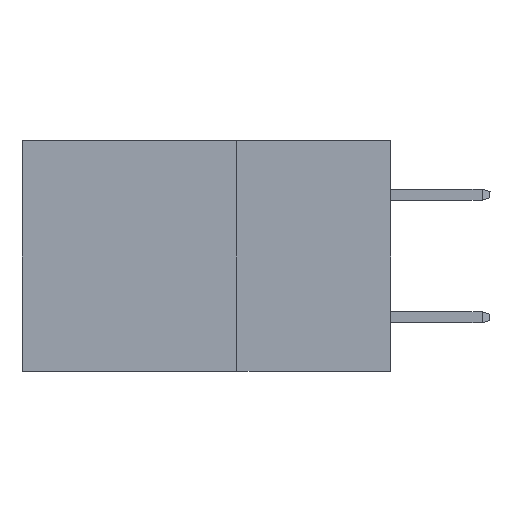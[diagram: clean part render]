
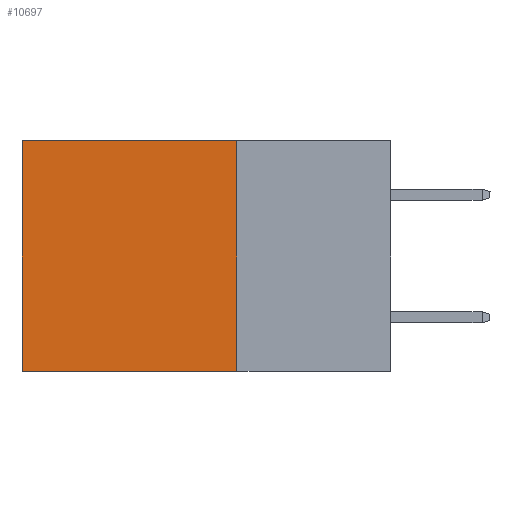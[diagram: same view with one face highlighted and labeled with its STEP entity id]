
A CAD part, left-side view. The second image highlights one B-rep face of the part: STEP entity #10697.
In plain terms, the highlighted planar face has unit normal (-1, 0, 0).
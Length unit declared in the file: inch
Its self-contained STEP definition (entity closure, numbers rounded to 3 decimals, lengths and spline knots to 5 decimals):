
#198 = CARTESIAN_POINT ( 'NONE',  ( 0.2875, 0.6, 0. ) ) ;
#1148 = EDGE_LOOP ( 'NONE', ( #4128, #6292, #8601, #3034 ) ) ;
#2045 = CARTESIAN_POINT ( 'NONE',  ( 0.2875, 0.25, -0.375 ) ) ;
#2134 = AXIS2_PLACEMENT_3D ( 'NONE', #2045, #3228, #10731 ) ;
#3034 = ORIENTED_EDGE ( 'NONE', *, *, #6800, .T. ) ;
#3228 = DIRECTION ( 'NONE',  ( 1., 0., 0. ) ) ;
#3261 = VERTEX_POINT ( 'NONE', #7658 ) ;
#3534 = DIRECTION ( 'NONE',  ( 0., 0., -1. ) ) ;
#3937 = EDGE_CURVE ( 'NONE', #3261, #6011, #5675, .T. ) ;
#4128 = ORIENTED_EDGE ( 'NONE', *, *, #8604, .T. ) ;
#4240 = CARTESIAN_POINT ( 'NONE',  ( 0.2875, 0.25, -0.375 ) ) ;
#4877 = VECTOR ( 'NONE', #5059, 39.37008 ) ;
#5059 = DIRECTION ( 'NONE',  ( 0., 1., 0. ) ) ;
#5675 = LINE ( 'NONE', #11109, #6325 ) ;
#6011 = VERTEX_POINT ( 'NONE', #12541 ) ;
#6292 = ORIENTED_EDGE ( 'NONE', *, *, #11213, .F. ) ;
#6325 = VECTOR ( 'NONE', #12013, 39.37008 ) ;
#6518 = VERTEX_POINT ( 'NONE', #7511 ) ;
#6800 = EDGE_CURVE ( 'NONE', #3261, #7610, #13750, .T. ) ;
#7511 = CARTESIAN_POINT ( 'NONE',  ( 0.2875, 0.6, -0.375 ) ) ;
#7610 = VERTEX_POINT ( 'NONE', #198 ) ;
#7630 = LINE ( 'NONE', #4240, #12957 ) ;
#7658 = CARTESIAN_POINT ( 'NONE',  ( 0.2875, 0.25, 0. ) ) ;
#8601 = ORIENTED_EDGE ( 'NONE', *, *, #3937, .F. ) ;
#8604 = EDGE_CURVE ( 'NONE', #7610, #6518, #13059, .T. ) ;
#9238 = CARTESIAN_POINT ( 'NONE',  ( 0.2875, 0.25, 0. ) ) ;
#9430 = FACE_OUTER_BOUND ( 'NONE', #1148, .T. ) ;
#9800 = DIRECTION ( 'NONE',  ( 0., 1., 0. ) ) ;
#9932 = CARTESIAN_POINT ( 'NONE',  ( 0.2875, 0.6, -0.375 ) ) ;
#10534 = PLANE ( 'NONE',  #2134 ) ;
#10697 = ADVANCED_FACE ( 'NONE', ( #9430 ), #10534, .F. ) ;
#10731 = DIRECTION ( 'NONE',  ( 0., 0., -1. ) ) ;
#10860 = VECTOR ( 'NONE', #3534, 39.37008 ) ;
#11109 = CARTESIAN_POINT ( 'NONE',  ( 0.2875, 0.25, -0.375 ) ) ;
#11213 = EDGE_CURVE ( 'NONE', #6011, #6518, #7630, .T. ) ;
#12013 = DIRECTION ( 'NONE',  ( 0., 0., -1. ) ) ;
#12541 = CARTESIAN_POINT ( 'NONE',  ( 0.2875, 0.25, -0.375 ) ) ;
#12957 = VECTOR ( 'NONE', #9800, 39.37008 ) ;
#13059 = LINE ( 'NONE', #9932, #10860 ) ;
#13750 = LINE ( 'NONE', #9238, #4877 ) ;
